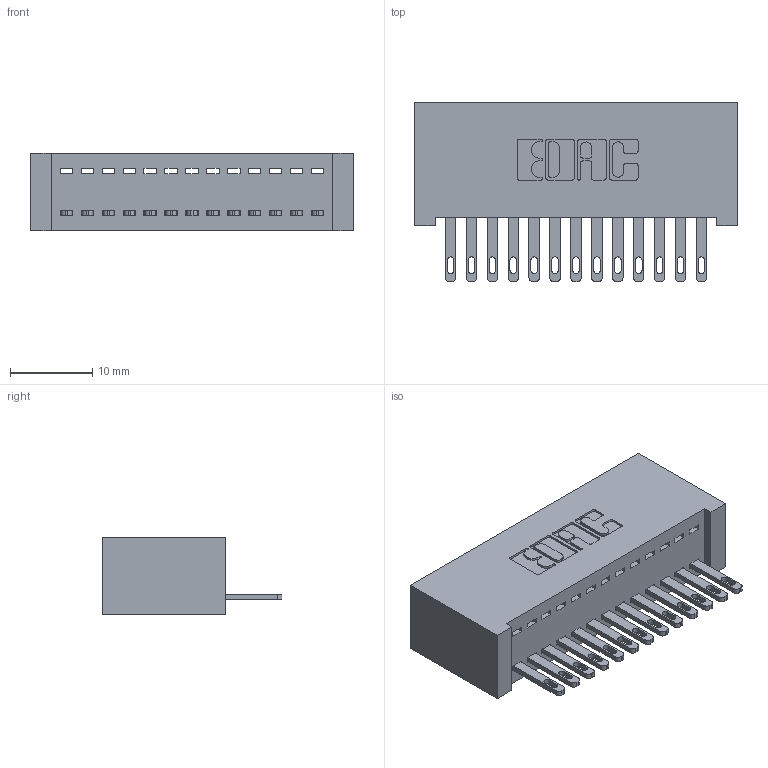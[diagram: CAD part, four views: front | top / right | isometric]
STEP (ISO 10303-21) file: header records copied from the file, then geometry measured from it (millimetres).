
FILE_DESCRIPTION (( 'STEP AP203' ), '1' );
FILE_NAME ('342-013-500-101.STEP', '2018-08-10T16:02:35', ( '' ), ( '' ), 'SwSTEP 2.0', 'SolidWorks 2016', '' );
FILE_SCHEMA (( 'CONFIG_CONTROL_DESIGN' ));
Length unit declared in the file: inch
Products named in the file (3): 342 Part_Lugless; 345-292-001_345-293-100; 342-013-500-101
Assembly tree (14 placements, depth 2):
  342-013-500-101
    342 Part_Lugless
    345-292-001_345-293-100  x13
Bounding box: 39.27 x 21.85 x 9.4 mm (x, y, z)
Volume: 3753.3 mm3; surface area: 5318.9 mm2
Topology: 14 solids, 14 shells, 804 faces, 2459 edges, 1638 vertices
Faces by surface type: plane 530, cylinder 274
Entity records: 11219 total; most frequent: CARTESIAN_POINT 1945, ORIENTED_EDGE 1894, DIRECTION 1693, EDGE_CURVE 947, LINE 823, VECTOR 823, VERTEX_POINT 630, AXIS2_PLACEMENT_3D 435
